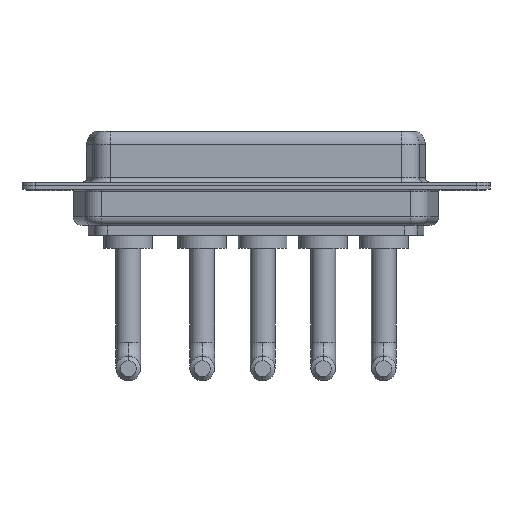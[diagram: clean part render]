
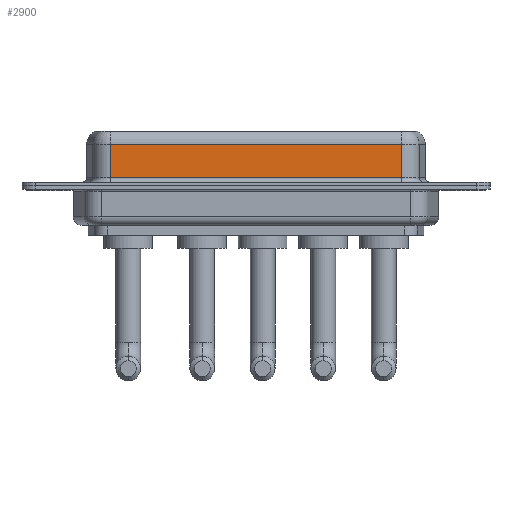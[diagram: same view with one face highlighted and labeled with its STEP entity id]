
A CAD part, front view. The second image highlights one B-rep face of the part: STEP entity #2900.
In plain terms, the highlighted planar face has unit normal (0, -1, 0).
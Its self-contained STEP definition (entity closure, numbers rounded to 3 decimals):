
#365 = DIRECTION ( 'NONE',  ( 0., 0., -1. ) ) ;
#402 = CARTESIAN_POINT ( 'NONE',  ( 40.037, -3.95, 4.65 ) ) ;
#595 = LINE ( 'NONE', #10827, #3861 ) ;
#1016 = LINE ( 'NONE', #1083, #9421 ) ;
#1083 = CARTESIAN_POINT ( 'NONE',  ( 40.037, -3.95, 0.9 ) ) ;
#1150 = VERTEX_POINT ( 'NONE', #8970 ) ;
#1170 = ORIENTED_EDGE ( 'NONE', *, *, #10026, .F. ) ;
#1348 = LINE ( 'NONE', #6276, #2829 ) ;
#2058 = EDGE_CURVE ( 'NONE', #5283, #1150, #1016, .T. ) ;
#2621 = AXIS2_PLACEMENT_3D ( 'NONE', #9279, #8330, #7488 ) ;
#2637 = EDGE_CURVE ( 'NONE', #7406, #4895, #5541, .T. ) ;
#2723 = CARTESIAN_POINT ( 'NONE',  ( 7.013, -3.95, 4.65 ) ) ;
#2829 = VECTOR ( 'NONE', #365, 1000. ) ;
#2900 = ADVANCED_FACE ( 'NONE', ( #4124 ), #8430, .F. ) ;
#3238 = CARTESIAN_POINT ( 'NONE',  ( 7.013, -3.95, 0.9 ) ) ;
#3509 = ORIENTED_EDGE ( 'NONE', *, *, #2058, .T. ) ;
#3861 = VECTOR ( 'NONE', #7325, 1000. ) ;
#4124 = FACE_OUTER_BOUND ( 'NONE', #5382, .T. ) ;
#4895 = VERTEX_POINT ( 'NONE', #2723 ) ;
#5283 = VERTEX_POINT ( 'NONE', #3238 ) ;
#5382 = EDGE_LOOP ( 'NONE', ( #1170, #8469, #5769, #3509 ) ) ;
#5434 = DIRECTION ( 'NONE',  ( 1., 0., 0. ) ) ;
#5541 = LINE ( 'NONE', #402, #10399 ) ;
#5769 = ORIENTED_EDGE ( 'NONE', *, *, #8989, .T. ) ;
#6276 = CARTESIAN_POINT ( 'NONE',  ( 7.013, -3.95, 6.4 ) ) ;
#7325 = DIRECTION ( 'NONE',  ( 0., 0., -1. ) ) ;
#7406 = VERTEX_POINT ( 'NONE', #10761 ) ;
#7488 = DIRECTION ( 'NONE',  ( 0., 0., 1. ) ) ;
#8065 = DIRECTION ( 'NONE',  ( -1., 0., 0. ) ) ;
#8330 = DIRECTION ( 'NONE',  ( 0., 1., 0. ) ) ;
#8430 = PLANE ( 'NONE',  #2621 ) ;
#8469 = ORIENTED_EDGE ( 'NONE', *, *, #2637, .T. ) ;
#8970 = CARTESIAN_POINT ( 'NONE',  ( 40.037, -3.95, 0.9 ) ) ;
#8989 = EDGE_CURVE ( 'NONE', #4895, #5283, #1348, .T. ) ;
#9279 = CARTESIAN_POINT ( 'NONE',  ( 40.037, -3.95, 6.4 ) ) ;
#9421 = VECTOR ( 'NONE', #5434, 1000. ) ;
#10026 = EDGE_CURVE ( 'NONE', #7406, #1150, #595, .T. ) ;
#10399 = VECTOR ( 'NONE', #8065, 1000. ) ;
#10761 = CARTESIAN_POINT ( 'NONE',  ( 40.037, -3.95, 4.65 ) ) ;
#10827 = CARTESIAN_POINT ( 'NONE',  ( 40.037, -3.95, 6.4 ) ) ;
